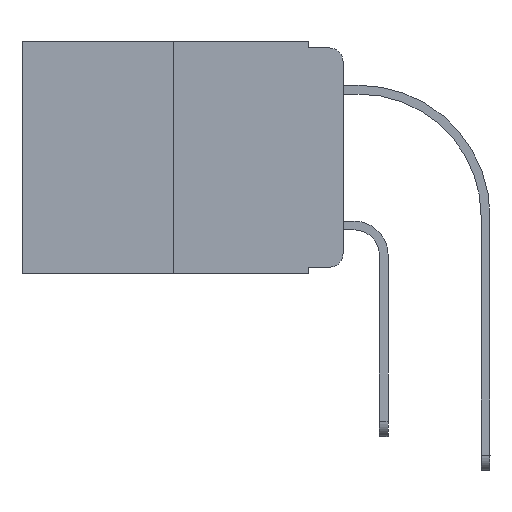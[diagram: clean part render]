
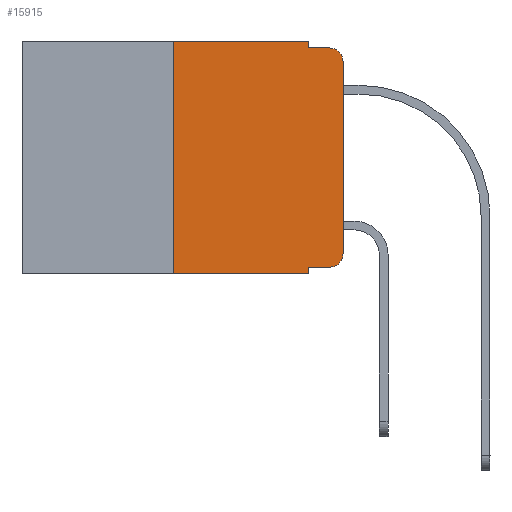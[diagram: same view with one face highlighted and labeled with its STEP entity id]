
A CAD part, left-side view. The second image highlights one B-rep face of the part: STEP entity #15915.
In plain terms, the highlighted planar face has unit normal (-1, 0, 0).
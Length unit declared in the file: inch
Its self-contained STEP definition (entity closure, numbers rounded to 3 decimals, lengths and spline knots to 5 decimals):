
#18 = LINE ( 'NONE', #14197, #16627 ) ;
#125 = VECTOR ( 'NONE', #10426, 39.37008 ) ;
#273 = CARTESIAN_POINT ( 'NONE',  ( 0., 0.051, -0.333 ) ) ;
#537 = LINE ( 'NONE', #6170, #17678 ) ;
#564 = FACE_OUTER_BOUND ( 'NONE', #2666, .T. ) ;
#593 = DIRECTION ( 'NONE',  ( 0., 0., 1. ) ) ;
#629 = CARTESIAN_POINT ( 'NONE',  ( 0., 0.051, -0.333 ) ) ;
#652 = LINE ( 'NONE', #6379, #125 ) ;
#1459 = EDGE_CURVE ( 'NONE', #10539, #2991, #12668, .T. ) ;
#1511 = VERTEX_POINT ( 'NONE', #1849 ) ;
#1828 = CARTESIAN_POINT ( 'NONE',  ( 0., 0.25, 0. ) ) ;
#1849 = CARTESIAN_POINT ( 'NONE',  ( 0., 0.25, -0.343 ) ) ;
#1893 = VECTOR ( 'NONE', #7204, 39.37008 ) ;
#2197 = VERTEX_POINT ( 'NONE', #5558 ) ;
#2601 = VECTOR ( 'NONE', #6828, 39.37008 ) ;
#2666 = EDGE_LOOP ( 'NONE', ( #10799, #7554, #3976, #2972, #17006, #8994, #14854, #17848, #6479, #4278 ) ) ;
#2972 = ORIENTED_EDGE ( 'NONE', *, *, #15877, .F. ) ;
#2991 = VERTEX_POINT ( 'NONE', #15556 ) ;
#3215 = CARTESIAN_POINT ( 'NONE',  ( 0., 0.473, 0. ) ) ;
#3368 = EDGE_CURVE ( 'NONE', #2197, #5966, #5299, .T. ) ;
#3445 = CARTESIAN_POINT ( 'NONE',  ( 0., 0.02, -0.03 ) ) ;
#3472 = LINE ( 'NONE', #9189, #9633 ) ;
#3917 = CARTESIAN_POINT ( 'NONE',  ( 0., 0.02, -0.01 ) ) ;
#3976 = ORIENTED_EDGE ( 'NONE', *, *, #8423, .F. ) ;
#4278 = ORIENTED_EDGE ( 'NONE', *, *, #1459, .T. ) ;
#5144 = LINE ( 'NONE', #629, #16983 ) ;
#5299 = CIRCLE ( 'NONE', #6192, 0.02 ) ;
#5558 = CARTESIAN_POINT ( 'NONE',  ( 0., 0., -0.03 ) ) ;
#5707 = CARTESIAN_POINT ( 'NONE',  ( 0., 0.473, -0.343 ) ) ;
#5858 = EDGE_CURVE ( 'NONE', #2991, #2197, #537, .T. ) ;
#5966 = VERTEX_POINT ( 'NONE', #3917 ) ;
#6170 = CARTESIAN_POINT ( 'NONE',  ( 0., 0., 0. ) ) ;
#6192 = AXIS2_PLACEMENT_3D ( 'NONE', #3445, #8035, #13759 ) ;
#6289 = PLANE ( 'NONE',  #10916 ) ;
#6379 = CARTESIAN_POINT ( 'NONE',  ( 0., 0.051, 0. ) ) ;
#6479 = ORIENTED_EDGE ( 'NONE', *, *, #14556, .T. ) ;
#6736 = CARTESIAN_POINT ( 'NONE',  ( 0., 0.473, 0. ) ) ;
#6828 = DIRECTION ( 'NONE',  ( 0., -1., 0. ) ) ;
#7112 = CARTESIAN_POINT ( 'NONE',  ( 0., 0.02, -0.313 ) ) ;
#7204 = DIRECTION ( 'NONE',  ( 0., -1., 0. ) ) ;
#7240 = VERTEX_POINT ( 'NONE', #7776 ) ;
#7554 = ORIENTED_EDGE ( 'NONE', *, *, #3368, .T. ) ;
#7776 = CARTESIAN_POINT ( 'NONE',  ( 0., 0.051, 0. ) ) ;
#8035 = DIRECTION ( 'NONE',  ( -1., 0., 0. ) ) ;
#8288 = VERTEX_POINT ( 'NONE', #273 ) ;
#8423 = EDGE_CURVE ( 'NONE', #10721, #5966, #3472, .T. ) ;
#8454 = VERTEX_POINT ( 'NONE', #16327 ) ;
#8745 = AXIS2_PLACEMENT_3D ( 'NONE', #7112, #12918, #12829 ) ;
#8925 = DIRECTION ( 'NONE',  ( 1., 0., 0. ) ) ;
#8994 = ORIENTED_EDGE ( 'NONE', *, *, #9357, .F. ) ;
#9087 = DIRECTION ( 'NONE',  ( 0., -1., 0. ) ) ;
#9189 = CARTESIAN_POINT ( 'NONE',  ( 0., 0.051, -0.01 ) ) ;
#9357 = EDGE_CURVE ( 'NONE', #1511, #8454, #10456, .T. ) ;
#9589 = EDGE_CURVE ( 'NONE', #8288, #14059, #18, .T. ) ;
#9633 = VECTOR ( 'NONE', #9087, 39.37008 ) ;
#9964 = DIRECTION ( 'NONE',  ( 0., 0., -1. ) ) ;
#10426 = DIRECTION ( 'NONE',  ( 0., 0., -1. ) ) ;
#10456 = LINE ( 'NONE', #1828, #13604 ) ;
#10539 = VERTEX_POINT ( 'NONE', #14319 ) ;
#10545 = CARTESIAN_POINT ( 'NONE',  ( 0., 0.051, -0.01 ) ) ;
#10721 = VERTEX_POINT ( 'NONE', #10545 ) ;
#10799 = ORIENTED_EDGE ( 'NONE', *, *, #5858, .T. ) ;
#10916 = AXIS2_PLACEMENT_3D ( 'NONE', #3215, #8925, #12005 ) ;
#11841 = EDGE_CURVE ( 'NONE', #1511, #14059, #15656, .T. ) ;
#12005 = DIRECTION ( 'NONE',  ( 0., 0., -1. ) ) ;
#12668 = CIRCLE ( 'NONE', #8745, 0.02 ) ;
#12829 = DIRECTION ( 'NONE',  ( 0., 0., -1. ) ) ;
#12918 = DIRECTION ( 'NONE',  ( -1., 0., 0. ) ) ;
#13604 = VECTOR ( 'NONE', #593, 39.37008 ) ;
#13759 = DIRECTION ( 'NONE',  ( 0., 0., -1. ) ) ;
#13869 = LINE ( 'NONE', #6736, #2601 ) ;
#14059 = VERTEX_POINT ( 'NONE', #16087 ) ;
#14197 = CARTESIAN_POINT ( 'NONE',  ( 0., 0.051, 0. ) ) ;
#14319 = CARTESIAN_POINT ( 'NONE',  ( 0., 0.02, -0.333 ) ) ;
#14556 = EDGE_CURVE ( 'NONE', #8288, #10539, #5144, .T. ) ;
#14716 = EDGE_CURVE ( 'NONE', #8454, #7240, #13869, .T. ) ;
#14854 = ORIENTED_EDGE ( 'NONE', *, *, #11841, .T. ) ;
#15556 = CARTESIAN_POINT ( 'NONE',  ( 0., 0., -0.313 ) ) ;
#15656 = LINE ( 'NONE', #5707, #1893 ) ;
#15877 = EDGE_CURVE ( 'NONE', #7240, #10721, #652, .T. ) ;
#15915 = ADVANCED_FACE ( 'NONE', ( #564 ), #6289, .F. ) ;
#16087 = CARTESIAN_POINT ( 'NONE',  ( 0., 0.051, -0.343 ) ) ;
#16327 = CARTESIAN_POINT ( 'NONE',  ( 0., 0.25, 0. ) ) ;
#16500 = DIRECTION ( 'NONE',  ( 0., 0., 1. ) ) ;
#16627 = VECTOR ( 'NONE', #9964, 39.37008 ) ;
#16983 = VECTOR ( 'NONE', #17826, 39.37008 ) ;
#17006 = ORIENTED_EDGE ( 'NONE', *, *, #14716, .F. ) ;
#17678 = VECTOR ( 'NONE', #16500, 39.37008 ) ;
#17826 = DIRECTION ( 'NONE',  ( 0., -1., 0. ) ) ;
#17848 = ORIENTED_EDGE ( 'NONE', *, *, #9589, .F. ) ;
